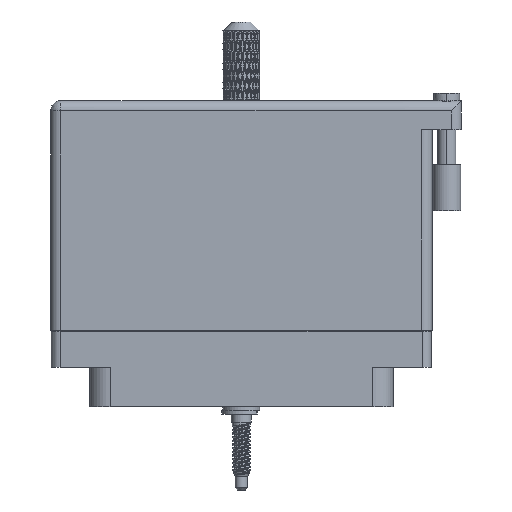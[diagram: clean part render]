
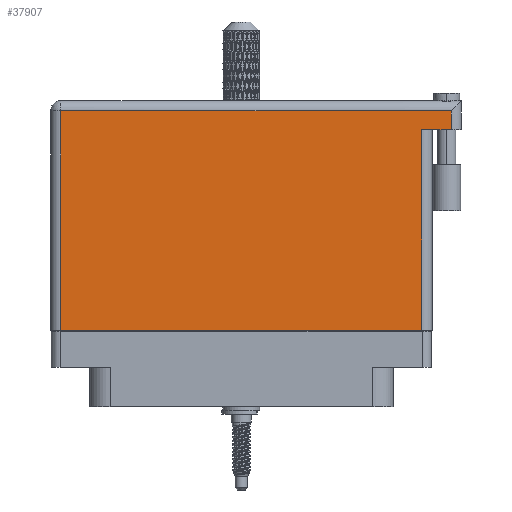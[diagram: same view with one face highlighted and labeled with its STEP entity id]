
A CAD part, front view. The second image highlights one B-rep face of the part: STEP entity #37907.
In plain terms, the highlighted face is planar.
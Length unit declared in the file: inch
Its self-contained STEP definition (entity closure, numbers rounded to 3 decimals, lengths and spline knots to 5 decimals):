
#1959 = CARTESIAN_POINT ( 'NONE',  ( 1.23, 1.269, 0.4495 ) ) ;
#2567 = ORIENTED_EDGE ( 'NONE', *, *, #69807, .T. ) ;
#3551 = VERTEX_POINT ( 'NONE', #1959 ) ;
#7892 = ORIENTED_EDGE ( 'NONE', *, *, #111155, .T. ) ;
#12368 = CARTESIAN_POINT ( 'NONE',  ( -1.3, 1.466, 0.4495 ) ) ;
#13748 = DIRECTION ( 'NONE',  ( 0., 1., 0. ) ) ;
#14335 = EDGE_CURVE ( 'NONE', #82309, #3551, #16653, .T. ) ;
#16653 = LINE ( 'NONE', #51066, #80630 ) ;
#17321 = CARTESIAN_POINT ( 'NONE',  ( -1.3, -0.1, 0.4495 ) ) ;
#18213 = CARTESIAN_POINT ( 'NONE',  ( 1.23, -0.1, 0.4495 ) ) ;
#19503 = LINE ( 'NONE', #17321, #68418 ) ;
#26065 = ORIENTED_EDGE ( 'NONE', *, *, #49432, .T. ) ;
#26522 = VERTEX_POINT ( 'NONE', #31187 ) ;
#26708 = VECTOR ( 'NONE', #93548, 39.37008 ) ;
#30188 = PLANE ( 'NONE',  #58937 ) ;
#31187 = CARTESIAN_POINT ( 'NONE',  ( -1.23, -0.1, 0.4495 ) ) ;
#33355 = ORIENTED_EDGE ( 'NONE', *, *, #48842, .T. ) ;
#33955 = CARTESIAN_POINT ( 'NONE',  ( 1.23, 1.269, 0.4495 ) ) ;
#37907 = ADVANCED_FACE ( 'NONE', ( #39090 ), #30188, .F. ) ;
#39090 = FACE_OUTER_BOUND ( 'NONE', #73706, .T. ) ;
#39679 = DIRECTION ( 'NONE',  ( 0., 0., -1. ) ) ;
#42273 = DIRECTION ( 'NONE',  ( 0., 1., 0. ) ) ;
#46470 = VERTEX_POINT ( 'NONE', #60866 ) ;
#46625 = CARTESIAN_POINT ( 'NONE',  ( -1.3, 1.396, 0.4495 ) ) ;
#48562 = DIRECTION ( 'NONE',  ( -1., 0., 0. ) ) ;
#48842 = EDGE_CURVE ( 'NONE', #46470, #105959, #84644, .T. ) ;
#49432 = EDGE_CURVE ( 'NONE', #26522, #104435, #19503, .T. ) ;
#51066 = CARTESIAN_POINT ( 'NONE',  ( 1.5, 1.269, 0.4495 ) ) ;
#52390 = VECTOR ( 'NONE', #13748, 39.37008 ) ;
#52826 = DIRECTION ( 'NONE',  ( -1., 0., 0. ) ) ;
#58937 = AXIS2_PLACEMENT_3D ( 'NONE', #12368, #39679, #48562 ) ;
#60627 = LINE ( 'NONE', #103420, #52390 ) ;
#60866 = CARTESIAN_POINT ( 'NONE',  ( 1.43, 1.396, 0.4495 ) ) ;
#67851 = LINE ( 'NONE', #33955, #79833 ) ;
#68286 = VECTOR ( 'NONE', #68938, 39.37008 ) ;
#68418 = VECTOR ( 'NONE', #83035, 39.37008 ) ;
#68938 = DIRECTION ( 'NONE',  ( 0., -1., 0. ) ) ;
#69807 = EDGE_CURVE ( 'NONE', #105959, #26522, #87917, .T. ) ;
#73706 = EDGE_LOOP ( 'NONE', ( #26065, #7892, #92036, #100344, #33355, #2567 ) ) ;
#79606 = CARTESIAN_POINT ( 'NONE',  ( -1.23, -0.1, 0.4495 ) ) ;
#79833 = VECTOR ( 'NONE', #42273, 39.37008 ) ;
#80630 = VECTOR ( 'NONE', #52826, 39.37008 ) ;
#82309 = VERTEX_POINT ( 'NONE', #84916 ) ;
#83035 = DIRECTION ( 'NONE',  ( 1., 0., 0. ) ) ;
#84644 = LINE ( 'NONE', #46625, #26708 ) ;
#84916 = CARTESIAN_POINT ( 'NONE',  ( 1.43, 1.269, 0.4495 ) ) ;
#87917 = LINE ( 'NONE', #79606, #68286 ) ;
#92036 = ORIENTED_EDGE ( 'NONE', *, *, #14335, .F. ) ;
#93548 = DIRECTION ( 'NONE',  ( -1., 0., 0. ) ) ;
#94091 = EDGE_CURVE ( 'NONE', #82309, #46470, #60627, .T. ) ;
#94211 = CARTESIAN_POINT ( 'NONE',  ( -1.23, 1.396, 0.4495 ) ) ;
#100344 = ORIENTED_EDGE ( 'NONE', *, *, #94091, .T. ) ;
#103420 = CARTESIAN_POINT ( 'NONE',  ( 1.43, 1.466, 0.4495 ) ) ;
#104435 = VERTEX_POINT ( 'NONE', #18213 ) ;
#105959 = VERTEX_POINT ( 'NONE', #94211 ) ;
#111155 = EDGE_CURVE ( 'NONE', #104435, #3551, #67851, .T. ) ;
